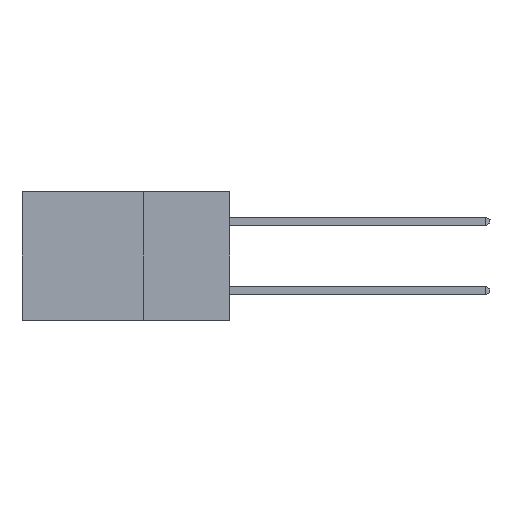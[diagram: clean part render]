
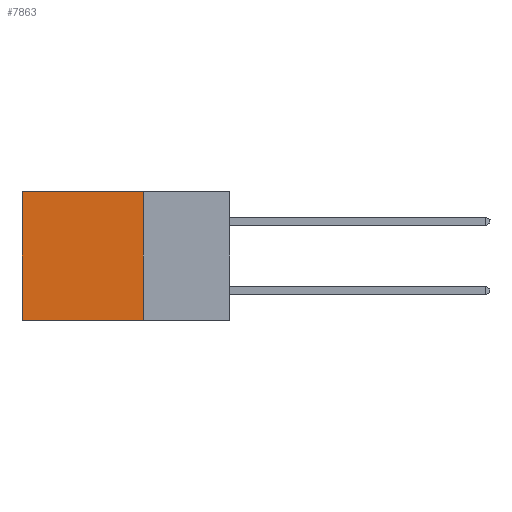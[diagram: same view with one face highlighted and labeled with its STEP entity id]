
A CAD part, left-side view. The second image highlights one B-rep face of the part: STEP entity #7863.
In plain terms, the highlighted planar face has unit normal (-1, 0, 0).
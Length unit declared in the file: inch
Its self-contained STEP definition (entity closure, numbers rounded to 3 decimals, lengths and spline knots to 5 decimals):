
#457 = EDGE_CURVE ( 'NONE', #10532, #7326, #1810, .T. ) ;
#554 = ORIENTED_EDGE ( 'NONE', *, *, #5532, .F. ) ;
#854 = LINE ( 'NONE', #18402, #18703 ) ;
#1076 = EDGE_CURVE ( 'NONE', #13444, #8556, #16190, .T. ) ;
#1810 = LINE ( 'NONE', #7047, #4557 ) ;
#2142 = CARTESIAN_POINT ( 'NONE',  ( 0.298, 0.25, 0. ) ) ;
#2801 = EDGE_LOOP ( 'NONE', ( #3293, #554, #4131, #18478 ) ) ;
#3293 = ORIENTED_EDGE ( 'NONE', *, *, #457, .T. ) ;
#4131 = ORIENTED_EDGE ( 'NONE', *, *, #1076, .F. ) ;
#4209 = EDGE_CURVE ( 'NONE', #13444, #10532, #854, .T. ) ;
#4557 = VECTOR ( 'NONE', #15878, 39.37008 ) ;
#4693 = VECTOR ( 'NONE', #8393, 39.37008 ) ;
#4900 = CARTESIAN_POINT ( 'NONE',  ( 0.298, 0.6, 0. ) ) ;
#5092 = DIRECTION ( 'NONE',  ( 0., 0., -1. ) ) ;
#5532 = EDGE_CURVE ( 'NONE', #8556, #7326, #12441, .T. ) ;
#5965 = CARTESIAN_POINT ( 'NONE',  ( 0.298, 0.25, -0.37 ) ) ;
#6244 = CARTESIAN_POINT ( 'NONE',  ( 0.298, 0.25, 0. ) ) ;
#6769 = CARTESIAN_POINT ( 'NONE',  ( 0.298, 0.25, -0.37 ) ) ;
#7047 = CARTESIAN_POINT ( 'NONE',  ( 0.298, 0.6, 0. ) ) ;
#7326 = VERTEX_POINT ( 'NONE', #11179 ) ;
#7863 = ADVANCED_FACE ( 'NONE', ( #12160 ), #8349, .F. ) ;
#8349 = PLANE ( 'NONE',  #18306 ) ;
#8393 = DIRECTION ( 'NONE',  ( 0., 1., 0. ) ) ;
#8556 = VERTEX_POINT ( 'NONE', #5965 ) ;
#9654 = DIRECTION ( 'NONE',  ( 0., 1., 0. ) ) ;
#10532 = VERTEX_POINT ( 'NONE', #4900 ) ;
#11179 = CARTESIAN_POINT ( 'NONE',  ( 0.298, 0.6, -0.37 ) ) ;
#12160 = FACE_OUTER_BOUND ( 'NONE', #2801, .T. ) ;
#12288 = VECTOR ( 'NONE', #13803, 39.37008 ) ;
#12441 = LINE ( 'NONE', #6769, #4693 ) ;
#13300 = DIRECTION ( 'NONE',  ( 1., 0., 0. ) ) ;
#13444 = VERTEX_POINT ( 'NONE', #6244 ) ;
#13803 = DIRECTION ( 'NONE',  ( 0., 0., -1. ) ) ;
#14258 = CARTESIAN_POINT ( 'NONE',  ( 0.298, 0.25, 0. ) ) ;
#15878 = DIRECTION ( 'NONE',  ( 0., 0., -1. ) ) ;
#16190 = LINE ( 'NONE', #2142, #12288 ) ;
#18306 = AXIS2_PLACEMENT_3D ( 'NONE', #14258, #13300, #5092 ) ;
#18402 = CARTESIAN_POINT ( 'NONE',  ( 0.298, 0.25, 0. ) ) ;
#18478 = ORIENTED_EDGE ( 'NONE', *, *, #4209, .T. ) ;
#18703 = VECTOR ( 'NONE', #9654, 39.37008 ) ;
